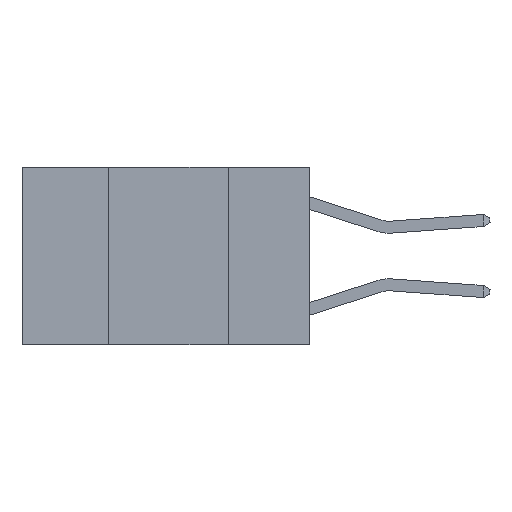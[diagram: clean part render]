
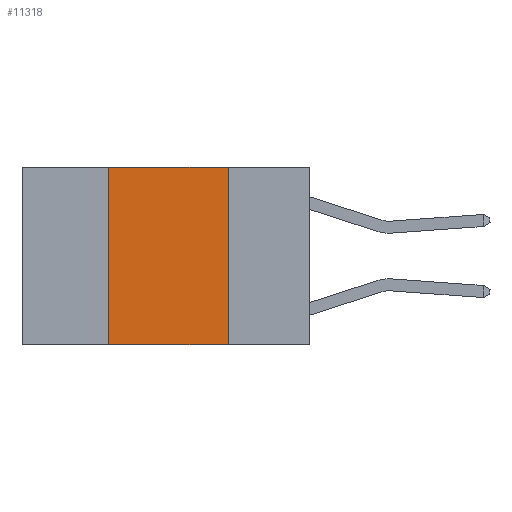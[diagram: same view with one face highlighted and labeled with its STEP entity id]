
A CAD part, left-side view. The second image highlights one B-rep face of the part: STEP entity #11318.
In plain terms, the highlighted planar face has unit normal (-1, 0, 0).
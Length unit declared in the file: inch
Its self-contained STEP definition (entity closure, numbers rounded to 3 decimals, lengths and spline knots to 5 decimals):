
#1030 = DIRECTION ( 'NONE',  ( 0., 0., 1. ) ) ;
#1109 = ORIENTED_EDGE ( 'NONE', *, *, #5616, .F. ) ;
#1224 = CARTESIAN_POINT ( 'NONE',  ( 0., 0.6, 0. ) ) ;
#1603 = VERTEX_POINT ( 'NONE', #15139 ) ;
#2237 = ORIENTED_EDGE ( 'NONE', *, *, #7968, .T. ) ;
#2303 = FACE_OUTER_BOUND ( 'NONE', #4119, .T. ) ;
#2897 = EDGE_CURVE ( 'NONE', #8085, #3637, #7808, .T. ) ;
#3075 = VECTOR ( 'NONE', #13239, 39.37008 ) ;
#3388 = CARTESIAN_POINT ( 'NONE',  ( 0., 0.17, 0. ) ) ;
#3637 = VERTEX_POINT ( 'NONE', #3388 ) ;
#3714 = CARTESIAN_POINT ( 'NONE',  ( 0., 0.6, 0. ) ) ;
#3820 = LINE ( 'NONE', #9249, #15840 ) ;
#3879 = DIRECTION ( 'NONE',  ( 0., 0., -1. ) ) ;
#4119 = EDGE_LOOP ( 'NONE', ( #10847, #8710, #1109, #2237 ) ) ;
#5120 = CARTESIAN_POINT ( 'NONE',  ( 0., 0.42, 0. ) ) ;
#5616 = EDGE_CURVE ( 'NONE', #1603, #8085, #6487, .T. ) ;
#6487 = LINE ( 'NONE', #5120, #14482 ) ;
#7808 = LINE ( 'NONE', #1224, #17170 ) ;
#7968 = EDGE_CURVE ( 'NONE', #1603, #14275, #9223, .T. ) ;
#8085 = VERTEX_POINT ( 'NONE', #13911 ) ;
#8526 = AXIS2_PLACEMENT_3D ( 'NONE', #3714, #8972, #3879 ) ;
#8710 = ORIENTED_EDGE ( 'NONE', *, *, #2897, .F. ) ;
#8887 = PLANE ( 'NONE',  #8526 ) ;
#8972 = DIRECTION ( 'NONE',  ( 1., 0., 0. ) ) ;
#9127 = CARTESIAN_POINT ( 'NONE',  ( 0., 0.6, -0.37 ) ) ;
#9212 = DIRECTION ( 'NONE',  ( 0., -1., 0. ) ) ;
#9223 = LINE ( 'NONE', #9127, #3075 ) ;
#9249 = CARTESIAN_POINT ( 'NONE',  ( 0., 0.17, 0. ) ) ;
#10847 = ORIENTED_EDGE ( 'NONE', *, *, #15189, .F. ) ;
#11318 = ADVANCED_FACE ( 'NONE', ( #2303 ), #8887, .F. ) ;
#13239 = DIRECTION ( 'NONE',  ( 0., -1., 0. ) ) ;
#13911 = CARTESIAN_POINT ( 'NONE',  ( 0., 0.42, 0. ) ) ;
#14275 = VERTEX_POINT ( 'NONE', #15835 ) ;
#14482 = VECTOR ( 'NONE', #1030, 39.37008 ) ;
#15139 = CARTESIAN_POINT ( 'NONE',  ( 0., 0.42, -0.37 ) ) ;
#15189 = EDGE_CURVE ( 'NONE', #3637, #14275, #3820, .T. ) ;
#15835 = CARTESIAN_POINT ( 'NONE',  ( 0., 0.17, -0.37 ) ) ;
#15840 = VECTOR ( 'NONE', #17098, 39.37008 ) ;
#17098 = DIRECTION ( 'NONE',  ( 0., 0., -1. ) ) ;
#17170 = VECTOR ( 'NONE', #9212, 39.37008 ) ;
